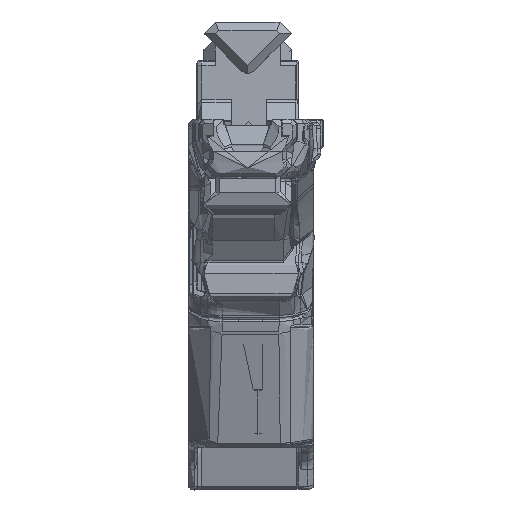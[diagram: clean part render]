
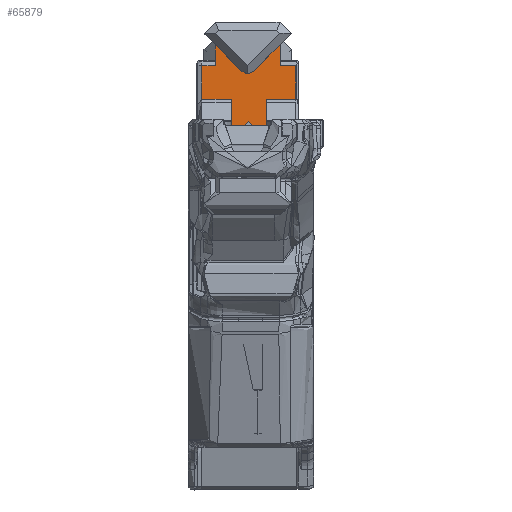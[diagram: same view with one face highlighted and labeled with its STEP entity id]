
A CAD part, left-side view. The second image highlights one B-rep face of the part: STEP entity #65879.
In plain terms, the highlighted planar face has unit normal (-1, 0, 0).
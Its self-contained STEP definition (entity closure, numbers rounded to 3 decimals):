
#414 = ORIENTED_EDGE ( 'NONE', *, *, #23223, .T. ) ;
#1355 = VERTEX_POINT ( 'NONE', #48531 ) ;
#1765 = ORIENTED_EDGE ( 'NONE', *, *, #56464, .F. ) ;
#1847 = FACE_OUTER_BOUND ( 'NONE', #70603, .T. ) ;
#2838 = CARTESIAN_POINT ( 'NONE',  ( 72.964, 77.944, 17.979 ) ) ;
#3135 = CIRCLE ( 'NONE', #12986, 2. ) ;
#3185 = DIRECTION ( 'NONE',  ( 0., 0., -1. ) ) ;
#4532 = ORIENTED_EDGE ( 'NONE', *, *, #23703, .T. ) ;
#5614 = VECTOR ( 'NONE', #68525, 1000. ) ;
#5772 = DIRECTION ( 'NONE',  ( 1., 0., 0. ) ) ;
#6304 = CARTESIAN_POINT ( 'NONE',  ( 72.964, 81.274, 12.919 ) ) ;
#6339 = VERTEX_POINT ( 'NONE', #8751 ) ;
#6838 = CARTESIAN_POINT ( 'NONE',  ( 72.964, 65.607, 4.76 ) ) ;
#6987 = LINE ( 'NONE', #24712, #11551 ) ;
#7337 = VECTOR ( 'NONE', #17670, 1000. ) ;
#7440 = VERTEX_POINT ( 'NONE', #73460 ) ;
#8043 = DIRECTION ( 'NONE',  ( 0., -1., 0. ) ) ;
#8451 = EDGE_CURVE ( 'NONE', #40730, #7440, #3135, .T. ) ;
#8656 = CARTESIAN_POINT ( 'NONE',  ( 72.964, 59.509, 20.744 ) ) ;
#8751 = CARTESIAN_POINT ( 'NONE',  ( 72.964, 62.271, 17.979 ) ) ;
#9277 = VERTEX_POINT ( 'NONE', #52129 ) ;
#9359 = ORIENTED_EDGE ( 'NONE', *, *, #74059, .F. ) ;
#10551 = LINE ( 'NONE', #46752, #65951 ) ;
#11551 = VECTOR ( 'NONE', #14301, 1000. ) ;
#12986 = AXIS2_PLACEMENT_3D ( 'NONE', #29648, #5772, #16555 ) ;
#13847 = DIRECTION ( 'NONE',  ( 0., -1., 0. ) ) ;
#14301 = DIRECTION ( 'NONE',  ( 0., -0.707, -0.707 ) ) ;
#14398 = ORIENTED_EDGE ( 'NONE', *, *, #54127, .T. ) ;
#14438 = LINE ( 'NONE', #50260, #53100 ) ;
#14559 = LINE ( 'NONE', #56925, #5614 ) ;
#15624 = EDGE_CURVE ( 'NONE', #56555, #1355, #57735, .T. ) ;
#15629 = VECTOR ( 'NONE', #34520, 1000. ) ;
#16555 = DIRECTION ( 'NONE',  ( 0., 0., 1. ) ) ;
#16723 = VERTEX_POINT ( 'NONE', #6838 ) ;
#17670 = DIRECTION ( 'NONE',  ( 0., 0., -1. ) ) ;
#17829 = EDGE_CURVE ( 'NONE', #7440, #56555, #10551, .T. ) ;
#19008 = VECTOR ( 'NONE', #72281, 1000. ) ;
#19559 = VECTOR ( 'NONE', #54437, 1000. ) ;
#20192 = LINE ( 'NONE', #43329, #49906 ) ;
#20389 = VERTEX_POINT ( 'NONE', #56562 ) ;
#20773 = CARTESIAN_POINT ( 'NONE',  ( 72.964, 58.414, -17.335 ) ) ;
#20933 = ORIENTED_EDGE ( 'NONE', *, *, #17829, .T. ) ;
#21700 = VERTEX_POINT ( 'NONE', #39456 ) ;
#22519 = CARTESIAN_POINT ( 'NONE',  ( 72.964, 70.114, 4.76 ) ) ;
#22635 = DIRECTION ( 'NONE',  ( 0., 1., 0. ) ) ;
#22638 = VERTEX_POINT ( 'NONE', #53622 ) ;
#23223 = EDGE_CURVE ( 'NONE', #66048, #21700, #27276, .T. ) ;
#23703 = EDGE_CURVE ( 'NONE', #1355, #44381, #53690, .T. ) ;
#23822 = CARTESIAN_POINT ( 'NONE',  ( 72.964, 58.414, 12.919 ) ) ;
#24712 = CARTESIAN_POINT ( 'NONE',  ( 72.964, 71.805, 1.307 ) ) ;
#24747 = ORIENTED_EDGE ( 'NONE', *, *, #49604, .T. ) ;
#25376 = DIRECTION ( 'NONE',  ( 0., 1., 0. ) ) ;
#26322 = LINE ( 'NONE', #38259, #71882 ) ;
#26521 = VERTEX_POINT ( 'NONE', #53054 ) ;
#27025 = ORIENTED_EDGE ( 'NONE', *, *, #29548, .F. ) ;
#27276 = LINE ( 'NONE', #43486, #38070 ) ;
#27669 = CARTESIAN_POINT ( 'NONE',  ( 72.964, 62.279, 17.979 ) ) ;
#27946 = LINE ( 'NONE', #22519, #44696 ) ;
#29548 = EDGE_CURVE ( 'NONE', #50065, #44381, #20192, .T. ) ;
#29648 = CARTESIAN_POINT ( 'NONE',  ( 72.964, 70.109, 12.973 ) ) ;
#31798 = VERTEX_POINT ( 'NONE', #53727 ) ;
#34309 = DIRECTION ( 'NONE',  ( 0., 0., 1. ) ) ;
#34520 = DIRECTION ( 'NONE',  ( 0., 0., -1. ) ) ;
#34615 = ORIENTED_EDGE ( 'NONE', *, *, #64058, .F. ) ;
#35047 = VECTOR ( 'NONE', #22635, 1000. ) ;
#38070 = VECTOR ( 'NONE', #8043, 1000. ) ;
#38257 = ORIENTED_EDGE ( 'NONE', *, *, #71368, .T. ) ;
#38259 = CARTESIAN_POINT ( 'NONE',  ( 72.964, 74.08, -13.142 ) ) ;
#38286 = EDGE_CURVE ( 'NONE', #56146, #31798, #62044, .T. ) ;
#39456 = CARTESIAN_POINT ( 'NONE',  ( 72.964, 74.08, 4.76 ) ) ;
#40252 = DIRECTION ( 'NONE',  ( 0., -1., 0. ) ) ;
#40328 = CARTESIAN_POINT ( 'NONE',  ( 72.964, 81.274, 4.76 ) ) ;
#40730 = VERTEX_POINT ( 'NONE', #68129 ) ;
#40961 = DIRECTION ( 'NONE',  ( 0., 0.707, 0.707 ) ) ;
#41539 = ORIENTED_EDGE ( 'NONE', *, *, #8451, .T. ) ;
#42959 = LINE ( 'NONE', #8656, #54802 ) ;
#43327 = CARTESIAN_POINT ( 'NONE',  ( 72.964, 67.882, 1.307 ) ) ;
#43329 = CARTESIAN_POINT ( 'NONE',  ( 72.964, 77.891, 12.919 ) ) ;
#43486 = CARTESIAN_POINT ( 'NONE',  ( 72.964, 70.114, 4.76 ) ) ;
#44096 = DIRECTION ( 'NONE',  ( 0., -1., 0. ) ) ;
#44381 = VERTEX_POINT ( 'NONE', #56414 ) ;
#44696 = VECTOR ( 'NONE', #40252, 1000. ) ;
#45465 = ORIENTED_EDGE ( 'NONE', *, *, #55441, .F. ) ;
#46752 = CARTESIAN_POINT ( 'NONE',  ( 72.964, 70.753, 10.788 ) ) ;
#47744 = DIRECTION ( 'NONE',  ( -1., 0., 0. ) ) ;
#48125 = CARTESIAN_POINT ( 'NONE',  ( 72.964, 70.114, 11.428 ) ) ;
#48531 = CARTESIAN_POINT ( 'NONE',  ( 72.964, 77.949, 17.979 ) ) ;
#48748 = DIRECTION ( 'NONE',  ( 0., -0.707, 0.707 ) ) ;
#49268 = CARTESIAN_POINT ( 'NONE',  ( 72.964, 62.274, 17.979 ) ) ;
#49292 = LINE ( 'NONE', #67449, #69620 ) ;
#49604 = EDGE_CURVE ( 'NONE', #21700, #26521, #26322, .T. ) ;
#49906 = VECTOR ( 'NONE', #66883, 1000. ) ;
#50065 = VERTEX_POINT ( 'NONE', #6304 ) ;
#50260 = CARTESIAN_POINT ( 'NONE',  ( 72.964, 77.891, 12.919 ) ) ;
#51661 = CARTESIAN_POINT ( 'NONE',  ( 72.964, 81.274, -17.335 ) ) ;
#52129 = CARTESIAN_POINT ( 'NONE',  ( 72.964, 69.844, -0.654 ) ) ;
#53054 = CARTESIAN_POINT ( 'NONE',  ( 72.964, 74.08, -4.891 ) ) ;
#53100 = VECTOR ( 'NONE', #44096, 1000. ) ;
#53622 = CARTESIAN_POINT ( 'NONE',  ( 72.964, 65.607, -4.891 ) ) ;
#53690 = LINE ( 'NONE', #72203, #19559 ) ;
#53727 = CARTESIAN_POINT ( 'NONE',  ( 72.964, 58.414, 4.76 ) ) ;
#54127 = EDGE_CURVE ( 'NONE', #26521, #9277, #72661, .T. ) ;
#54437 = DIRECTION ( 'NONE',  ( 0., 0., -1. ) ) ;
#54802 = VECTOR ( 'NONE', #48748, 1000. ) ;
#55441 = EDGE_CURVE ( 'NONE', #40730, #74208, #42959, .T. ) ;
#55579 = VECTOR ( 'NONE', #34309, 1000. ) ;
#56146 = VERTEX_POINT ( 'NONE', #23822 ) ;
#56414 = CARTESIAN_POINT ( 'NONE',  ( 72.964, 77.949, 12.919 ) ) ;
#56464 = EDGE_CURVE ( 'NONE', #6339, #20389, #14559, .T. ) ;
#56555 = VERTEX_POINT ( 'NONE', #2838 ) ;
#56562 = CARTESIAN_POINT ( 'NONE',  ( 72.964, 62.271, 12.919 ) ) ;
#56925 = CARTESIAN_POINT ( 'NONE',  ( 72.964, 62.271, 11.428 ) ) ;
#57511 = ORIENTED_EDGE ( 'NONE', *, *, #73800, .T. ) ;
#57735 = LINE ( 'NONE', #27669, #35047 ) ;
#57803 = LINE ( 'NONE', #64750, #7337 ) ;
#58539 = ORIENTED_EDGE ( 'NONE', *, *, #59281, .F. ) ;
#59281 = EDGE_CURVE ( 'NONE', #74208, #6339, #49292, .T. ) ;
#61128 = ORIENTED_EDGE ( 'NONE', *, *, #15624, .T. ) ;
#62044 = LINE ( 'NONE', #20773, #15629 ) ;
#64058 = EDGE_CURVE ( 'NONE', #20389, #56146, #14438, .T. ) ;
#64750 = CARTESIAN_POINT ( 'NONE',  ( 72.964, 65.607, -13.142 ) ) ;
#65879 = ADVANCED_FACE ( 'NONE', ( #1847 ), #72039, .T. ) ;
#65951 = VECTOR ( 'NONE', #40961, 1000. ) ;
#66048 = VERTEX_POINT ( 'NONE', #40328 ) ;
#66883 = DIRECTION ( 'NONE',  ( 0., -1., 0. ) ) ;
#67449 = CARTESIAN_POINT ( 'NONE',  ( 72.964, 70.114, 17.979 ) ) ;
#67950 = EDGE_CURVE ( 'NONE', #66048, #50065, #70161, .T. ) ;
#68129 = CARTESIAN_POINT ( 'NONE',  ( 72.964, 68.695, 11.558 ) ) ;
#68525 = DIRECTION ( 'NONE',  ( 0., 0., -1. ) ) ;
#68727 = ORIENTED_EDGE ( 'NONE', *, *, #38286, .F. ) ;
#69620 = VECTOR ( 'NONE', #13847, 1000. ) ;
#70161 = LINE ( 'NONE', #51661, #55579 ) ;
#70603 = EDGE_LOOP ( 'NONE', ( #75518, #414, #24747, #14398, #57511, #9359, #38257, #68727, #34615, #1765, #58539, #45465, #41539, #20933, #61128, #4532, #27025 ) ) ;
#71368 = EDGE_CURVE ( 'NONE', #16723, #31798, #27946, .T. ) ;
#71882 = VECTOR ( 'NONE', #3185, 1000. ) ;
#72039 = PLANE ( 'NONE',  #75266 ) ;
#72203 = CARTESIAN_POINT ( 'NONE',  ( 72.964, 77.949, 10.174 ) ) ;
#72281 = DIRECTION ( 'NONE',  ( 0., -0.707, 0.707 ) ) ;
#72661 = LINE ( 'NONE', #43327, #19008 ) ;
#73460 = CARTESIAN_POINT ( 'NONE',  ( 72.964, 71.524, 11.558 ) ) ;
#73800 = EDGE_CURVE ( 'NONE', #9277, #22638, #6987, .T. ) ;
#74059 = EDGE_CURVE ( 'NONE', #16723, #22638, #57803, .T. ) ;
#74208 = VERTEX_POINT ( 'NONE', #49268 ) ;
#75266 = AXIS2_PLACEMENT_3D ( 'NONE', #48125, #47744, #25376 ) ;
#75518 = ORIENTED_EDGE ( 'NONE', *, *, #67950, .F. ) ;
